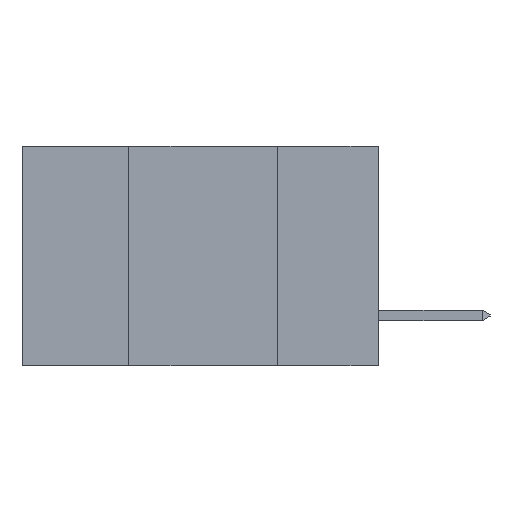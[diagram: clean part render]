
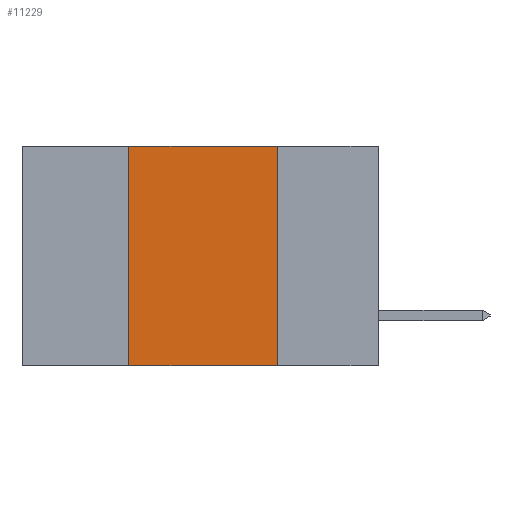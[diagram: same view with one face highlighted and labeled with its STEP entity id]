
A CAD part, left-side view. The second image highlights one B-rep face of the part: STEP entity #11229.
In plain terms, the highlighted planar face has unit normal (-1, 0, 0).
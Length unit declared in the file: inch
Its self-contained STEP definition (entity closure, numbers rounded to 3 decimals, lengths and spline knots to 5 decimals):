
#98 = DIRECTION ( 'NONE',  ( 0., -1., 0. ) ) ;
#340 = VERTEX_POINT ( 'NONE', #14639 ) ;
#383 = VERTEX_POINT ( 'NONE', #5536 ) ;
#1103 = ORIENTED_EDGE ( 'NONE', *, *, #1848, .F. ) ;
#1210 = CARTESIAN_POINT ( 'NONE',  ( 0., 0.6, 0. ) ) ;
#1383 = VECTOR ( 'NONE', #9538, 39.37008 ) ;
#1763 = CARTESIAN_POINT ( 'NONE',  ( 0., 0.6, 0. ) ) ;
#1848 = EDGE_CURVE ( 'NONE', #383, #14807, #7192, .T. ) ;
#2496 = VECTOR ( 'NONE', #2795, 39.37008 ) ;
#2795 = DIRECTION ( 'NONE',  ( 0., -1., 0. ) ) ;
#3411 = ORIENTED_EDGE ( 'NONE', *, *, #5189, .F. ) ;
#3543 = CARTESIAN_POINT ( 'NONE',  ( 0., 0.6, -0.37 ) ) ;
#3614 = VECTOR ( 'NONE', #14930, 39.37008 ) ;
#4338 = ORIENTED_EDGE ( 'NONE', *, *, #4367, .F. ) ;
#4367 = EDGE_CURVE ( 'NONE', #14234, #383, #7135, .T. ) ;
#5189 = EDGE_CURVE ( 'NONE', #340, #14234, #13955, .T. ) ;
#5536 = CARTESIAN_POINT ( 'NONE',  ( 0., 0.17, 0. ) ) ;
#5886 = AXIS2_PLACEMENT_3D ( 'NONE', #1763, #6696, #14758 ) ;
#6013 = EDGE_CURVE ( 'NONE', #340, #14807, #12303, .T. ) ;
#6696 = DIRECTION ( 'NONE',  ( 1., 0., 0. ) ) ;
#6795 = CARTESIAN_POINT ( 'NONE',  ( 0., 0.42, 0. ) ) ;
#7135 = LINE ( 'NONE', #1210, #9504 ) ;
#7192 = LINE ( 'NONE', #8529, #3614 ) ;
#8529 = CARTESIAN_POINT ( 'NONE',  ( 0., 0.17, -0.37 ) ) ;
#9504 = VECTOR ( 'NONE', #98, 39.37008 ) ;
#9538 = DIRECTION ( 'NONE',  ( 0., 0., 1. ) ) ;
#11229 = ADVANCED_FACE ( 'NONE', ( #14645 ), #12431, .F. ) ;
#11667 = EDGE_LOOP ( 'NONE', ( #1103, #4338, #3411, #14318 ) ) ;
#12303 = LINE ( 'NONE', #3543, #2496 ) ;
#12431 = PLANE ( 'NONE',  #5886 ) ;
#13955 = LINE ( 'NONE', #14368, #1383 ) ;
#14234 = VERTEX_POINT ( 'NONE', #6795 ) ;
#14318 = ORIENTED_EDGE ( 'NONE', *, *, #6013, .T. ) ;
#14368 = CARTESIAN_POINT ( 'NONE',  ( 0., 0.42, -0.37 ) ) ;
#14639 = CARTESIAN_POINT ( 'NONE',  ( 0., 0.42, -0.37 ) ) ;
#14645 = FACE_OUTER_BOUND ( 'NONE', #11667, .T. ) ;
#14758 = DIRECTION ( 'NONE',  ( 0., 0., -1. ) ) ;
#14807 = VERTEX_POINT ( 'NONE', #14923 ) ;
#14923 = CARTESIAN_POINT ( 'NONE',  ( 0., 0.17, -0.37 ) ) ;
#14930 = DIRECTION ( 'NONE',  ( 0., 0., -1. ) ) ;
